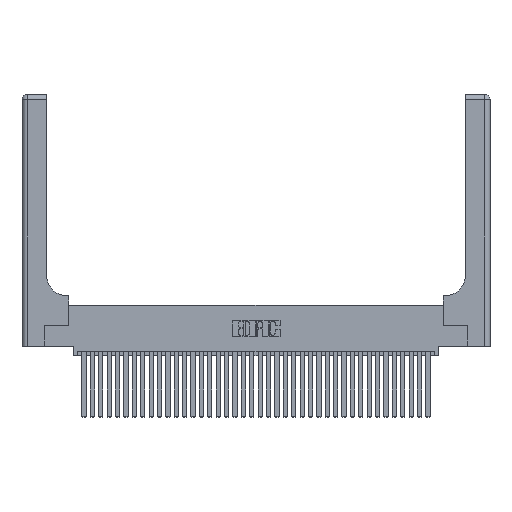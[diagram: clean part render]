
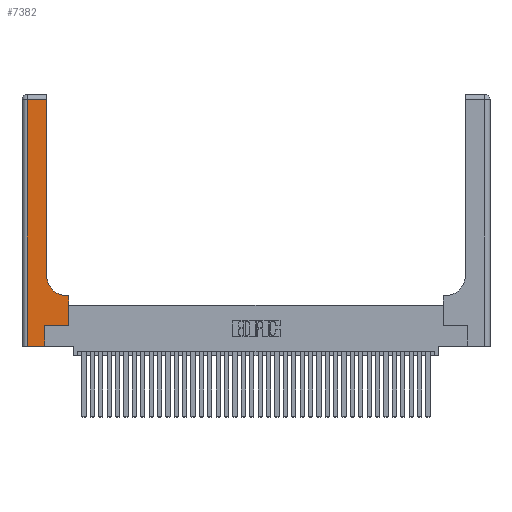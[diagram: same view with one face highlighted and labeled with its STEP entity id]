
A CAD part, top view. The second image highlights one B-rep face of the part: STEP entity #7382.
In plain terms, the highlighted planar face has unit normal (0, 0, 1).
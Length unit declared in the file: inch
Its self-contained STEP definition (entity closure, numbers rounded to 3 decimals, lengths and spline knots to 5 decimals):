
#430 = ORIENTED_EDGE ( 'NONE', *, *, #18710, .T. ) ;
#1192 = VECTOR ( 'NONE', #26668, 39.37008 ) ;
#1587 = CARTESIAN_POINT ( 'NONE',  ( 0.269, 0.25, 0.37 ) ) ;
#1995 = AXIS2_PLACEMENT_3D ( 'NONE', #12599, #10700, #33714 ) ;
#3982 = ORIENTED_EDGE ( 'NONE', *, *, #21868, .T. ) ;
#4023 = CARTESIAN_POINT ( 'NONE',  ( 0.2915, 2.94, 0.37 ) ) ;
#4042 = VECTOR ( 'NONE', #20820, 39.37008 ) ;
#4808 = CARTESIAN_POINT ( 'NONE',  ( 0.2915, 0.6, 0.37 ) ) ;
#5982 = ORIENTED_EDGE ( 'NONE', *, *, #32670, .T. ) ;
#6253 = VERTEX_POINT ( 'NONE', #37525 ) ;
#6730 = ORIENTED_EDGE ( 'NONE', *, *, #12927, .T. ) ;
#7382 = ADVANCED_FACE ( 'NONE', ( #31811 ), #9677, .F. ) ;
#7694 = LINE ( 'NONE', #1587, #21963 ) ;
#8218 = CARTESIAN_POINT ( 'NONE',  ( 0.06, 2.94, 0.37 ) ) ;
#8877 = LINE ( 'NONE', #38029, #11641 ) ;
#8979 = VERTEX_POINT ( 'NONE', #30904 ) ;
#9073 = DIRECTION ( 'NONE',  ( 1., 0., 0. ) ) ;
#9413 = CARTESIAN_POINT ( 'NONE',  ( 0.2915, 3., 0.37 ) ) ;
#9677 = PLANE ( 'NONE',  #1995 ) ;
#10700 = DIRECTION ( 'NONE',  ( 0., 0., -1. ) ) ;
#10873 = LINE ( 'NONE', #9413, #1192 ) ;
#10954 = LINE ( 'NONE', #24439, #36260 ) ;
#11641 = VECTOR ( 'NONE', #35168, 39.37008 ) ;
#11914 = DIRECTION ( 'NONE',  ( 0., -1., 0. ) ) ;
#12262 = LINE ( 'NONE', #12397, #4042 ) ;
#12320 = VERTEX_POINT ( 'NONE', #31905 ) ;
#12360 = EDGE_CURVE ( 'NONE', #32006, #30395, #10954, .T. ) ;
#12397 = CARTESIAN_POINT ( 'NONE',  ( 0.269, 0., 0.37 ) ) ;
#12599 = CARTESIAN_POINT ( 'NONE',  ( 0., 3., 0.37 ) ) ;
#12927 = EDGE_CURVE ( 'NONE', #31105, #32006, #7694, .T. ) ;
#13410 = EDGE_CURVE ( 'NONE', #8979, #20465, #10873, .T. ) ;
#13555 = LINE ( 'NONE', #32461, #20486 ) ;
#13570 = AXIS2_PLACEMENT_3D ( 'NONE', #24013, #24143, #33000 ) ;
#14514 = ORIENTED_EDGE ( 'NONE', *, *, #28110, .T. ) ;
#15243 = ORIENTED_EDGE ( 'NONE', *, *, #12360, .T. ) ;
#16938 = CIRCLE ( 'NONE', #13570, 0.25 ) ;
#17825 = CARTESIAN_POINT ( 'NONE',  ( 0.06, 3., 0.37 ) ) ;
#17962 = VERTEX_POINT ( 'NONE', #33674 ) ;
#18710 = EDGE_CURVE ( 'NONE', #30395, #12320, #35899, .T. ) ;
#18969 = CARTESIAN_POINT ( 'NONE',  ( 0.269, 0.25, 0.37 ) ) ;
#19987 = DIRECTION ( 'NONE',  ( 1., 0., 0. ) ) ;
#20465 = VERTEX_POINT ( 'NONE', #4023 ) ;
#20486 = VECTOR ( 'NONE', #9073, 39.37008 ) ;
#20820 = DIRECTION ( 'NONE',  ( 0., 1., 0. ) ) ;
#21868 = EDGE_CURVE ( 'NONE', #6253, #17962, #13555, .T. ) ;
#21963 = VECTOR ( 'NONE', #19987, 39.37008 ) ;
#23549 = VERTEX_POINT ( 'NONE', #8218 ) ;
#24013 = CARTESIAN_POINT ( 'NONE',  ( 0.5415, 0.85, 0.37 ) ) ;
#24143 = DIRECTION ( 'NONE',  ( 0., 0., -1. ) ) ;
#24439 = CARTESIAN_POINT ( 'NONE',  ( 0.5585, 0.25, 0.37 ) ) ;
#24986 = ORIENTED_EDGE ( 'NONE', *, *, #13410, .T. ) ;
#25812 = VECTOR ( 'NONE', #11914, 39.37008 ) ;
#26668 = DIRECTION ( 'NONE',  ( 0., 1., 0. ) ) ;
#27622 = CARTESIAN_POINT ( 'NONE',  ( 0.5585, 0.6, 0.37 ) ) ;
#28047 = VECTOR ( 'NONE', #31382, 39.37008 ) ;
#28110 = EDGE_CURVE ( 'NONE', #20465, #23549, #8877, .T. ) ;
#28111 = EDGE_LOOP ( 'NONE', ( #24986, #14514, #35141, #3982, #31516, #6730, #15243, #430, #5982 ) ) ;
#28544 = DIRECTION ( 'NONE',  ( 0., 1., 0. ) ) ;
#29469 = CARTESIAN_POINT ( 'NONE',  ( 0.5585, 0.25, 0.37 ) ) ;
#29475 = EDGE_CURVE ( 'NONE', #23549, #6253, #30328, .T. ) ;
#30328 = LINE ( 'NONE', #17825, #25812 ) ;
#30395 = VERTEX_POINT ( 'NONE', #27622 ) ;
#30904 = CARTESIAN_POINT ( 'NONE',  ( 0.2915, 0.85, 0.37 ) ) ;
#31105 = VERTEX_POINT ( 'NONE', #18969 ) ;
#31382 = DIRECTION ( 'NONE',  ( -1., 0., 0. ) ) ;
#31516 = ORIENTED_EDGE ( 'NONE', *, *, #32656, .T. ) ;
#31811 = FACE_OUTER_BOUND ( 'NONE', #28111, .T. ) ;
#31905 = CARTESIAN_POINT ( 'NONE',  ( 0.5415, 0.6, 0.37 ) ) ;
#32006 = VERTEX_POINT ( 'NONE', #29469 ) ;
#32461 = CARTESIAN_POINT ( 'NONE',  ( 0., 0., 0.37 ) ) ;
#32656 = EDGE_CURVE ( 'NONE', #17962, #31105, #12262, .T. ) ;
#32670 = EDGE_CURVE ( 'NONE', #12320, #8979, #16938, .T. ) ;
#33000 = DIRECTION ( 'NONE',  ( 1., 0., 0. ) ) ;
#33674 = CARTESIAN_POINT ( 'NONE',  ( 0.269, 0., 0.37 ) ) ;
#33714 = DIRECTION ( 'NONE',  ( -1., 0., 0. ) ) ;
#35141 = ORIENTED_EDGE ( 'NONE', *, *, #29475, .T. ) ;
#35168 = DIRECTION ( 'NONE',  ( -1., 0., 0. ) ) ;
#35899 = LINE ( 'NONE', #4808, #28047 ) ;
#36260 = VECTOR ( 'NONE', #28544, 39.37008 ) ;
#37525 = CARTESIAN_POINT ( 'NONE',  ( 0.06, 0., 0.37 ) ) ;
#38029 = CARTESIAN_POINT ( 'NONE',  ( 0., 2.94, 0.37 ) ) ;
